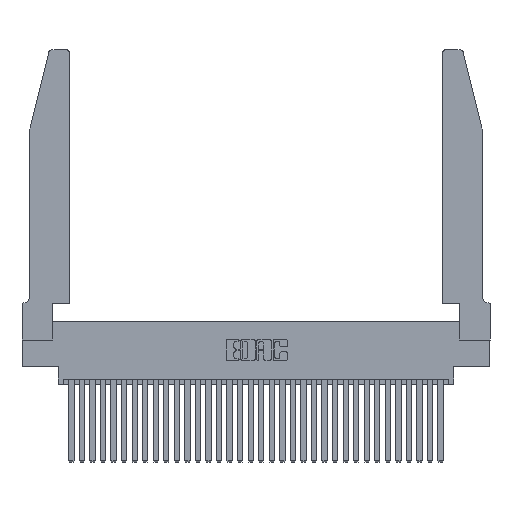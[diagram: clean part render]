
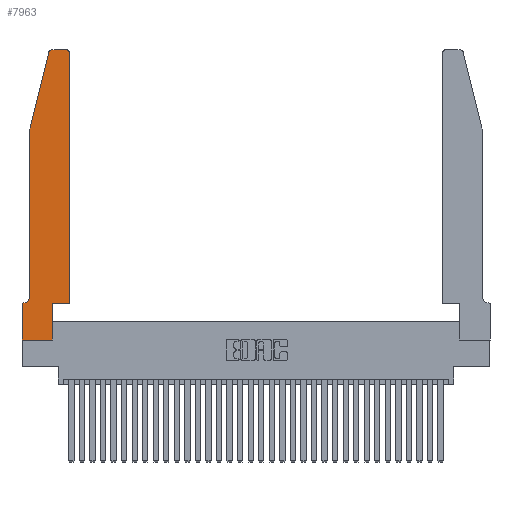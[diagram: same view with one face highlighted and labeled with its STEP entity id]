
A CAD part, top view. The second image highlights one B-rep face of the part: STEP entity #7963.
In plain terms, the highlighted planar face has unit normal (0, 0, 1).
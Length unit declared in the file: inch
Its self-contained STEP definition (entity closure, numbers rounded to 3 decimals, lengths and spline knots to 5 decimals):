
#517 = DIRECTION ( 'NONE',  ( 1., 0., 0. ) ) ;
#939 = VECTOR ( 'NONE', #2680, 39.37008 ) ;
#1395 = VERTEX_POINT ( 'NONE', #23338 ) ;
#1578 = VECTOR ( 'NONE', #23475, 39.37008 ) ;
#1618 = ORIENTED_EDGE ( 'NONE', *, *, #13043, .T. ) ;
#1724 = ORIENTED_EDGE ( 'NONE', *, *, #19055, .T. ) ;
#2593 = DIRECTION ( 'NONE',  ( -1., 0., 0. ) ) ;
#2609 = ORIENTED_EDGE ( 'NONE', *, *, #18556, .T. ) ;
#2673 = VERTEX_POINT ( 'NONE', #10006 ) ;
#2680 = DIRECTION ( 'NONE',  ( 0., -1., 0. ) ) ;
#2881 = EDGE_CURVE ( 'NONE', #2958, #4861, #11264, .T. ) ;
#2958 = VERTEX_POINT ( 'NONE', #16640 ) ;
#3266 = ORIENTED_EDGE ( 'NONE', *, *, #8365, .T. ) ;
#3653 = ORIENTED_EDGE ( 'NONE', *, *, #2881, .T. ) ;
#3946 = VECTOR ( 'NONE', #517, 39.37008 ) ;
#4633 = FACE_OUTER_BOUND ( 'NONE', #15596, .T. ) ;
#4719 = EDGE_CURVE ( 'NONE', #20936, #2958, #6298, .T. ) ;
#4861 = VERTEX_POINT ( 'NONE', #10622 ) ;
#6136 = DIRECTION ( 'NONE',  ( 1., 0., 0. ) ) ;
#6298 = LINE ( 'NONE', #32163, #28760 ) ;
#6656 = ORIENTED_EDGE ( 'NONE', *, *, #4719, .T. ) ;
#7456 = DIRECTION ( 'NONE',  ( 0., 0., 1. ) ) ;
#7677 = LINE ( 'NONE', #29523, #13802 ) ;
#7948 = ORIENTED_EDGE ( 'NONE', *, *, #25075, .T. ) ;
#7963 = ADVANCED_FACE ( 'NONE', ( #4633 ), #22346, .T. ) ;
#8365 = EDGE_CURVE ( 'NONE', #25346, #31339, #25848, .T. ) ;
#8761 = CARTESIAN_POINT ( 'NONE',  ( 0., 0.35, 0.37 ) ) ;
#9219 = ORIENTED_EDGE ( 'NONE', *, *, #19989, .T. ) ;
#10006 = CARTESIAN_POINT ( 'NONE',  ( 0.4505, 0.35, 0.37 ) ) ;
#10387 = AXIS2_PLACEMENT_3D ( 'NONE', #29722, #22093, #6136 ) ;
#10622 = CARTESIAN_POINT ( 'NONE',  ( 0.2865, 0., 0.37 ) ) ;
#10662 = EDGE_CURVE ( 'NONE', #19378, #20936, #7677, .T. ) ;
#10841 = CARTESIAN_POINT ( 'NONE',  ( 0.4505, 2.72, 0.37 ) ) ;
#11264 = LINE ( 'NONE', #16139, #3946 ) ;
#12323 = AXIS2_PLACEMENT_3D ( 'NONE', #17166, #7456, #23659 ) ;
#13043 = EDGE_CURVE ( 'NONE', #4861, #15526, #28242, .T. ) ;
#13187 = CARTESIAN_POINT ( 'NONE',  ( 0.4505, 0.35, 0.37 ) ) ;
#13539 = CARTESIAN_POINT ( 'NONE',  ( 0.0755, 2., 0.37 ) ) ;
#13802 = VECTOR ( 'NONE', #16522, 39.37008 ) ;
#14252 = DIRECTION ( 'NONE',  ( 0., -1., 0. ) ) ;
#14602 = CARTESIAN_POINT ( 'NONE',  ( 0.4205, 2.75, 0.37 ) ) ;
#15008 = LINE ( 'NONE', #13187, #1578 ) ;
#15526 = VERTEX_POINT ( 'NONE', #28115 ) ;
#15596 = EDGE_LOOP ( 'NONE', ( #1724, #25178, #3266, #25534, #22672, #22196, #6656, #3653, #1618, #2609, #7948, #9219 ) ) ;
#15647 = CARTESIAN_POINT ( 'NONE',  ( 0.0755, 2., 0.37 ) ) ;
#15888 = CARTESIAN_POINT ( 'NONE',  ( 0.0055, 0.42, 0.37 ) ) ;
#16139 = CARTESIAN_POINT ( 'NONE',  ( 0., 0., 0.37 ) ) ;
#16428 = CIRCLE ( 'NONE', #18059, 0.07 ) ;
#16522 = DIRECTION ( 'NONE',  ( -1., 0., 0. ) ) ;
#16640 = CARTESIAN_POINT ( 'NONE',  ( 0., 0., 0.37 ) ) ;
#16982 = DIRECTION ( 'NONE',  ( 0., 0., 1. ) ) ;
#17166 = CARTESIAN_POINT ( 'NONE',  ( 0.4205, 2.72, 0.37 ) ) ;
#18059 = AXIS2_PLACEMENT_3D ( 'NONE', #15888, #31439, #2593 ) ;
#18069 = VERTEX_POINT ( 'NONE', #10841 ) ;
#18233 = VECTOR ( 'NONE', #20021, 39.37008 ) ;
#18303 = LINE ( 'NONE', #31616, #21637 ) ;
#18556 = EDGE_CURVE ( 'NONE', #15526, #2673, #15008, .T. ) ;
#18924 = CARTESIAN_POINT ( 'NONE',  ( 0.0055, 0.35, 0.37 ) ) ;
#19055 = EDGE_CURVE ( 'NONE', #32188, #1395, #33381, .T. ) ;
#19240 = VECTOR ( 'NONE', #32246, 39.37008 ) ;
#19378 = VERTEX_POINT ( 'NONE', #18924 ) ;
#19824 = CARTESIAN_POINT ( 'NONE',  ( 0.25487, 2.72718, 0.37 ) ) ;
#19989 = EDGE_CURVE ( 'NONE', #18069, #32188, #20214, .T. ) ;
#20021 = DIRECTION ( 'NONE',  ( -1., 0., 0. ) ) ;
#20121 = LINE ( 'NONE', #15647, #939 ) ;
#20214 = CIRCLE ( 'NONE', #12323, 0.03 ) ;
#20480 = DIRECTION ( 'NONE',  ( 1., 0., 0. ) ) ;
#20936 = VERTEX_POINT ( 'NONE', #24154 ) ;
#21523 = EDGE_CURVE ( 'NONE', #31339, #24524, #20121, .T. ) ;
#21637 = VECTOR ( 'NONE', #26613, 39.37008 ) ;
#22093 = DIRECTION ( 'NONE',  ( 0., 0., 1. ) ) ;
#22196 = ORIENTED_EDGE ( 'NONE', *, *, #10662, .T. ) ;
#22263 = CARTESIAN_POINT ( 'NONE',  ( 0.2865, 0.35, 0.37 ) ) ;
#22346 = PLANE ( 'NONE',  #33069 ) ;
#22672 = ORIENTED_EDGE ( 'NONE', *, *, #28885, .T. ) ;
#23338 = CARTESIAN_POINT ( 'NONE',  ( 0.284, 2.75, 0.37 ) ) ;
#23475 = DIRECTION ( 'NONE',  ( 1., 0., 0. ) ) ;
#23528 = CARTESIAN_POINT ( 'NONE',  ( 0.0755, 2., 0.37 ) ) ;
#23659 = DIRECTION ( 'NONE',  ( 1., 0., 0. ) ) ;
#24154 = CARTESIAN_POINT ( 'NONE',  ( 0., 0.35, 0.37 ) ) ;
#24524 = VERTEX_POINT ( 'NONE', #32079 ) ;
#24793 = DIRECTION ( 'NONE',  ( 0., 1., 0. ) ) ;
#25075 = EDGE_CURVE ( 'NONE', #2673, #18069, #18303, .T. ) ;
#25178 = ORIENTED_EDGE ( 'NONE', *, *, #25733, .T. ) ;
#25346 = VERTEX_POINT ( 'NONE', #19824 ) ;
#25534 = ORIENTED_EDGE ( 'NONE', *, *, #21523, .T. ) ;
#25733 = EDGE_CURVE ( 'NONE', #1395, #25346, #27259, .T. ) ;
#25848 = LINE ( 'NONE', #13539, #19240 ) ;
#26612 = VECTOR ( 'NONE', #24793, 39.37008 ) ;
#26613 = DIRECTION ( 'NONE',  ( 0., 1., 0. ) ) ;
#27259 = CIRCLE ( 'NONE', #10387, 0.03 ) ;
#28115 = CARTESIAN_POINT ( 'NONE',  ( 0.2865, 0.35, 0.37 ) ) ;
#28242 = LINE ( 'NONE', #22263, #26612 ) ;
#28760 = VECTOR ( 'NONE', #14252, 39.37008 ) ;
#28885 = EDGE_CURVE ( 'NONE', #24524, #19378, #16428, .T. ) ;
#29523 = CARTESIAN_POINT ( 'NONE',  ( 0.0755, 0.35, 0.37 ) ) ;
#29722 = CARTESIAN_POINT ( 'NONE',  ( 0.284, 2.72, 0.37 ) ) ;
#30748 = CARTESIAN_POINT ( 'NONE',  ( 0.2605, 2.75, 0.37 ) ) ;
#31339 = VERTEX_POINT ( 'NONE', #23528 ) ;
#31439 = DIRECTION ( 'NONE',  ( 0., 0., -1. ) ) ;
#31616 = CARTESIAN_POINT ( 'NONE',  ( 0.4505, 0.35, 0.37 ) ) ;
#32079 = CARTESIAN_POINT ( 'NONE',  ( 0.0755, 0.42, 0.37 ) ) ;
#32163 = CARTESIAN_POINT ( 'NONE',  ( 0., 0., 0.37 ) ) ;
#32188 = VERTEX_POINT ( 'NONE', #14602 ) ;
#32246 = DIRECTION ( 'NONE',  ( -0.239, -0.971, 0. ) ) ;
#33069 = AXIS2_PLACEMENT_3D ( 'NONE', #8761, #16982, #20480 ) ;
#33381 = LINE ( 'NONE', #30748, #18233 ) ;
